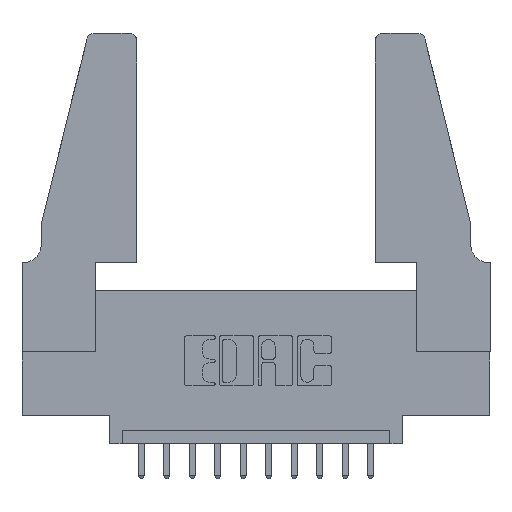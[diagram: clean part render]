
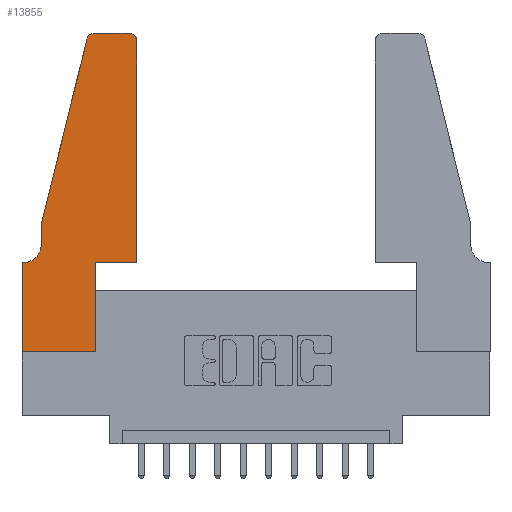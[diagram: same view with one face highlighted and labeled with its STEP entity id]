
A CAD part, top view. The second image highlights one B-rep face of the part: STEP entity #13855.
In plain terms, the highlighted planar face has unit normal (0, 0, 1).
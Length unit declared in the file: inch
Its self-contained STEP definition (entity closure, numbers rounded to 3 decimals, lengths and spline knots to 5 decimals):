
#460 = VECTOR ( 'NONE', #12160, 39.37008 ) ;
#470 = CARTESIAN_POINT ( 'NONE',  ( 0., 0., 0.37 ) ) ;
#586 = ORIENTED_EDGE ( 'NONE', *, *, #3600, .T. ) ;
#593 = VECTOR ( 'NONE', #7618, 39.37008 ) ;
#681 = DIRECTION ( 'NONE',  ( 0., 1., 0. ) ) ;
#688 = CARTESIAN_POINT ( 'NONE',  ( 0.0755, 0.42, 0.37 ) ) ;
#760 = DIRECTION ( 'NONE',  ( 1., 0., 0. ) ) ;
#1128 = EDGE_CURVE ( 'NONE', #5466, #6654, #9275, .T. ) ;
#1179 = LINE ( 'NONE', #6026, #4420 ) ;
#1376 = CARTESIAN_POINT ( 'NONE',  ( 0.0755, 0.35, 0.37 ) ) ;
#1446 = ORIENTED_EDGE ( 'NONE', *, *, #11722, .T. ) ;
#1787 = VERTEX_POINT ( 'NONE', #9013 ) ;
#2068 = VERTEX_POINT ( 'NONE', #4499 ) ;
#2127 = ORIENTED_EDGE ( 'NONE', *, *, #8203, .T. ) ;
#2245 = CARTESIAN_POINT ( 'NONE',  ( 0.2605, 1.25, 0.37 ) ) ;
#2305 = VECTOR ( 'NONE', #2533, 39.37008 ) ;
#2533 = DIRECTION ( 'NONE',  ( -0.239, -0.971, 0. ) ) ;
#2549 = CARTESIAN_POINT ( 'NONE',  ( 0., 0., 0.37 ) ) ;
#2722 = CARTESIAN_POINT ( 'NONE',  ( 0.2865, 0.35, 0.37 ) ) ;
#3010 = CARTESIAN_POINT ( 'NONE',  ( 0.25487, 1.22718, 0.37 ) ) ;
#3014 = VECTOR ( 'NONE', #4121, 39.37008 ) ;
#3072 = VERTEX_POINT ( 'NONE', #3852 ) ;
#3142 = EDGE_CURVE ( 'NONE', #2068, #4179, #4935, .T. ) ;
#3311 = LINE ( 'NONE', #11343, #5372 ) ;
#3361 = DIRECTION ( 'NONE',  ( 0., 0., 1. ) ) ;
#3511 = EDGE_CURVE ( 'NONE', #12056, #1787, #1179, .T. ) ;
#3600 = EDGE_CURVE ( 'NONE', #6004, #8059, #7489, .T. ) ;
#3769 = LINE ( 'NONE', #1376, #10086 ) ;
#3812 = CARTESIAN_POINT ( 'NONE',  ( 0.2865, 0.35, 0.37 ) ) ;
#3852 = CARTESIAN_POINT ( 'NONE',  ( 0., 0.35, 0.37 ) ) ;
#3941 = DIRECTION ( 'NONE',  ( 0., 0., 1. ) ) ;
#4000 = CARTESIAN_POINT ( 'NONE',  ( 0.0755, 0.5, 0.37 ) ) ;
#4121 = DIRECTION ( 'NONE',  ( 0., 1., 0. ) ) ;
#4179 = VERTEX_POINT ( 'NONE', #688 ) ;
#4199 = ORIENTED_EDGE ( 'NONE', *, *, #7963, .T. ) ;
#4420 = VECTOR ( 'NONE', #7085, 39.37008 ) ;
#4499 = CARTESIAN_POINT ( 'NONE',  ( 0.0755, 0.5, 0.37 ) ) ;
#4703 = DIRECTION ( 'NONE',  ( -1., 0., 0. ) ) ;
#4860 = VERTEX_POINT ( 'NONE', #7709 ) ;
#4935 = LINE ( 'NONE', #4000, #7844 ) ;
#5046 = DIRECTION ( 'NONE',  ( 0., 0., 1. ) ) ;
#5372 = VECTOR ( 'NONE', #6979, 39.37008 ) ;
#5428 = CARTESIAN_POINT ( 'NONE',  ( 0.4205, 1.25, 0.37 ) ) ;
#5466 = VERTEX_POINT ( 'NONE', #8700 ) ;
#5511 = CARTESIAN_POINT ( 'NONE',  ( 0., 0.35, 0.37 ) ) ;
#5533 = ORIENTED_EDGE ( 'NONE', *, *, #10323, .T. ) ;
#5548 = LINE ( 'NONE', #470, #593 ) ;
#5592 = CARTESIAN_POINT ( 'NONE',  ( 0.0755, 0.5, 0.37 ) ) ;
#5710 = CARTESIAN_POINT ( 'NONE',  ( 0.4505, 0.35, 0.37 ) ) ;
#6004 = VERTEX_POINT ( 'NONE', #9738 ) ;
#6026 = CARTESIAN_POINT ( 'NONE',  ( 0., 0., 0.37 ) ) ;
#6039 = VERTEX_POINT ( 'NONE', #5710 ) ;
#6488 = ORIENTED_EDGE ( 'NONE', *, *, #8234, .T. ) ;
#6540 = EDGE_CURVE ( 'NONE', #3072, #12056, #5548, .T. ) ;
#6654 = VERTEX_POINT ( 'NONE', #3010 ) ;
#6979 = DIRECTION ( 'NONE',  ( 1., 0., 0. ) ) ;
#7085 = DIRECTION ( 'NONE',  ( 1., 0., 0. ) ) ;
#7349 = AXIS2_PLACEMENT_3D ( 'NONE', #5511, #3361, #11010 ) ;
#7489 = CIRCLE ( 'NONE', #9037, 0.03 ) ;
#7618 = DIRECTION ( 'NONE',  ( 0., -1., 0. ) ) ;
#7709 = CARTESIAN_POINT ( 'NONE',  ( 0.0055, 0.35, 0.37 ) ) ;
#7844 = VECTOR ( 'NONE', #9621, 39.37008 ) ;
#7963 = EDGE_CURVE ( 'NONE', #8059, #5466, #12565, .T. ) ;
#8059 = VERTEX_POINT ( 'NONE', #5428 ) ;
#8154 = CARTESIAN_POINT ( 'NONE',  ( 0.0055, 0.42, 0.37 ) ) ;
#8203 = EDGE_CURVE ( 'NONE', #6039, #6004, #9151, .T. ) ;
#8234 = EDGE_CURVE ( 'NONE', #6654, #2068, #11396, .T. ) ;
#8318 = VERTEX_POINT ( 'NONE', #3812 ) ;
#8332 = ORIENTED_EDGE ( 'NONE', *, *, #3511, .T. ) ;
#8700 = CARTESIAN_POINT ( 'NONE',  ( 0.284, 1.25, 0.37 ) ) ;
#9013 = CARTESIAN_POINT ( 'NONE',  ( 0.2865, 0., 0.37 ) ) ;
#9037 = AXIS2_PLACEMENT_3D ( 'NONE', #11632, #3941, #12627 ) ;
#9151 = LINE ( 'NONE', #11672, #3014 ) ;
#9185 = ORIENTED_EDGE ( 'NONE', *, *, #6540, .T. ) ;
#9275 = CIRCLE ( 'NONE', #13130, 0.03 ) ;
#9306 = DIRECTION ( 'NONE',  ( -1., 0., 0. ) ) ;
#9435 = VECTOR ( 'NONE', #681, 39.37008 ) ;
#9593 = AXIS2_PLACEMENT_3D ( 'NONE', #8154, #12654, #9306 ) ;
#9621 = DIRECTION ( 'NONE',  ( 0., -1., 0. ) ) ;
#9738 = CARTESIAN_POINT ( 'NONE',  ( 0.4505, 1.22, 0.37 ) ) ;
#9876 = EDGE_CURVE ( 'NONE', #1787, #8318, #10487, .T. ) ;
#10086 = VECTOR ( 'NONE', #4703, 39.37008 ) ;
#10136 = ORIENTED_EDGE ( 'NONE', *, *, #3142, .T. ) ;
#10323 = EDGE_CURVE ( 'NONE', #4179, #4860, #12677, .T. ) ;
#10395 = EDGE_LOOP ( 'NONE', ( #4199, #11588, #6488, #10136, #5533, #1446, #9185, #8332, #11071, #11126, #2127, #586 ) ) ;
#10487 = LINE ( 'NONE', #2722, #9435 ) ;
#10515 = FACE_OUTER_BOUND ( 'NONE', #10395, .T. ) ;
#11010 = DIRECTION ( 'NONE',  ( 1., 0., 0. ) ) ;
#11071 = ORIENTED_EDGE ( 'NONE', *, *, #9876, .T. ) ;
#11126 = ORIENTED_EDGE ( 'NONE', *, *, #14014, .T. ) ;
#11343 = CARTESIAN_POINT ( 'NONE',  ( 0.4505, 0.35, 0.37 ) ) ;
#11396 = LINE ( 'NONE', #5592, #2305 ) ;
#11588 = ORIENTED_EDGE ( 'NONE', *, *, #1128, .T. ) ;
#11632 = CARTESIAN_POINT ( 'NONE',  ( 0.4205, 1.22, 0.37 ) ) ;
#11672 = CARTESIAN_POINT ( 'NONE',  ( 0.4505, 0.35, 0.37 ) ) ;
#11722 = EDGE_CURVE ( 'NONE', #4860, #3072, #3769, .T. ) ;
#11786 = CARTESIAN_POINT ( 'NONE',  ( 0.284, 1.22, 0.37 ) ) ;
#12056 = VERTEX_POINT ( 'NONE', #2549 ) ;
#12060 = PLANE ( 'NONE',  #7349 ) ;
#12160 = DIRECTION ( 'NONE',  ( -1., 0., 0. ) ) ;
#12565 = LINE ( 'NONE', #2245, #460 ) ;
#12627 = DIRECTION ( 'NONE',  ( 1., 0., 0. ) ) ;
#12654 = DIRECTION ( 'NONE',  ( 0., 0., -1. ) ) ;
#12677 = CIRCLE ( 'NONE', #9593, 0.07 ) ;
#13130 = AXIS2_PLACEMENT_3D ( 'NONE', #11786, #5046, #760 ) ;
#13855 = ADVANCED_FACE ( 'NONE', ( #10515 ), #12060, .T. ) ;
#14014 = EDGE_CURVE ( 'NONE', #8318, #6039, #3311, .T. ) ;
